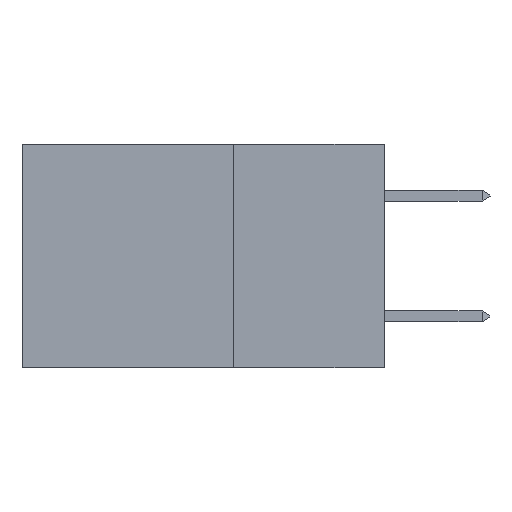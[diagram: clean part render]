
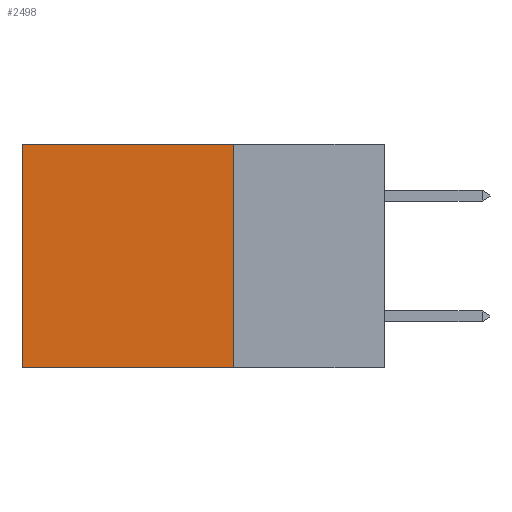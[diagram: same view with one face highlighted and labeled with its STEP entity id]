
A CAD part, left-side view. The second image highlights one B-rep face of the part: STEP entity #2498.
In plain terms, the highlighted planar face has unit normal (-1, 0, 0).
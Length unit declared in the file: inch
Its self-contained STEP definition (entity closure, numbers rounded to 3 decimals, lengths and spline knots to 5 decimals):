
#1070 = VERTEX_POINT ( 'NONE', #14658 ) ;
#1444 = VECTOR ( 'NONE', #14057, 39.37008 ) ;
#1606 = CARTESIAN_POINT ( 'NONE',  ( 0.2875, 0.25, 0. ) ) ;
#1841 = LINE ( 'NONE', #6230, #3970 ) ;
#2442 = CARTESIAN_POINT ( 'NONE',  ( 0.2875, 0.6, 0. ) ) ;
#2498 = ADVANCED_FACE ( 'NONE', ( #11926 ), #9006, .F. ) ;
#3970 = VECTOR ( 'NONE', #9326, 39.37008 ) ;
#5499 = VECTOR ( 'NONE', #16481, 39.37008 ) ;
#5885 = VERTEX_POINT ( 'NONE', #13125 ) ;
#5916 = VECTOR ( 'NONE', #14396, 39.37008 ) ;
#6230 = CARTESIAN_POINT ( 'NONE',  ( 0.2875, 0.25, 0. ) ) ;
#6400 = CARTESIAN_POINT ( 'NONE',  ( 0.2875, 0.6, -0.37 ) ) ;
#6767 = CARTESIAN_POINT ( 'NONE',  ( 0.2875, 0.25, -0.37 ) ) ;
#7463 = CARTESIAN_POINT ( 'NONE',  ( 0.2875, 0.25, 0. ) ) ;
#9006 = PLANE ( 'NONE',  #10867 ) ;
#9078 = EDGE_CURVE ( 'NONE', #18388, #17555, #14152, .T. ) ;
#9326 = DIRECTION ( 'NONE',  ( 0., 1., 0. ) ) ;
#9369 = EDGE_CURVE ( 'NONE', #5885, #18388, #10456, .T. ) ;
#9826 = LINE ( 'NONE', #2442, #5916 ) ;
#10448 = EDGE_CURVE ( 'NONE', #5885, #1070, #1841, .T. ) ;
#10456 = LINE ( 'NONE', #1606, #5499 ) ;
#10867 = AXIS2_PLACEMENT_3D ( 'NONE', #7463, #17854, #13392 ) ;
#11926 = FACE_OUTER_BOUND ( 'NONE', #14009, .T. ) ;
#12106 = ORIENTED_EDGE ( 'NONE', *, *, #9078, .F. ) ;
#12651 = CARTESIAN_POINT ( 'NONE',  ( 0.2875, 0.25, -0.37 ) ) ;
#12910 = EDGE_CURVE ( 'NONE', #1070, #17555, #9826, .T. ) ;
#13125 = CARTESIAN_POINT ( 'NONE',  ( 0.2875, 0.25, 0. ) ) ;
#13392 = DIRECTION ( 'NONE',  ( 0., 0., -1. ) ) ;
#13976 = ORIENTED_EDGE ( 'NONE', *, *, #12910, .T. ) ;
#14009 = EDGE_LOOP ( 'NONE', ( #13976, #12106, #19056, #16835 ) ) ;
#14057 = DIRECTION ( 'NONE',  ( 0., 1., 0. ) ) ;
#14152 = LINE ( 'NONE', #6767, #1444 ) ;
#14396 = DIRECTION ( 'NONE',  ( 0., 0., -1. ) ) ;
#14658 = CARTESIAN_POINT ( 'NONE',  ( 0.2875, 0.6, 0. ) ) ;
#16481 = DIRECTION ( 'NONE',  ( 0., 0., -1. ) ) ;
#16835 = ORIENTED_EDGE ( 'NONE', *, *, #10448, .T. ) ;
#17555 = VERTEX_POINT ( 'NONE', #6400 ) ;
#17854 = DIRECTION ( 'NONE',  ( 1., 0., 0. ) ) ;
#18388 = VERTEX_POINT ( 'NONE', #12651 ) ;
#19056 = ORIENTED_EDGE ( 'NONE', *, *, #9369, .F. ) ;
